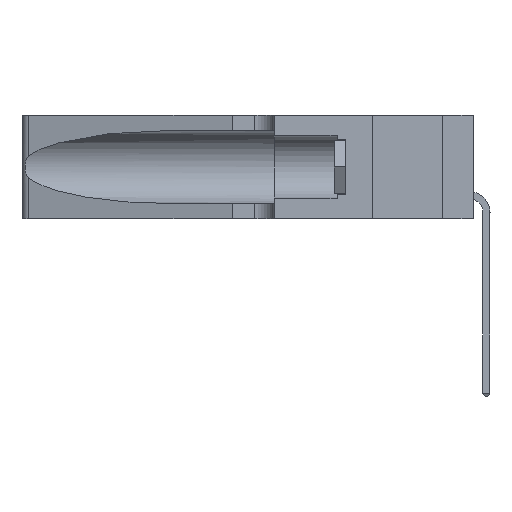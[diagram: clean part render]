
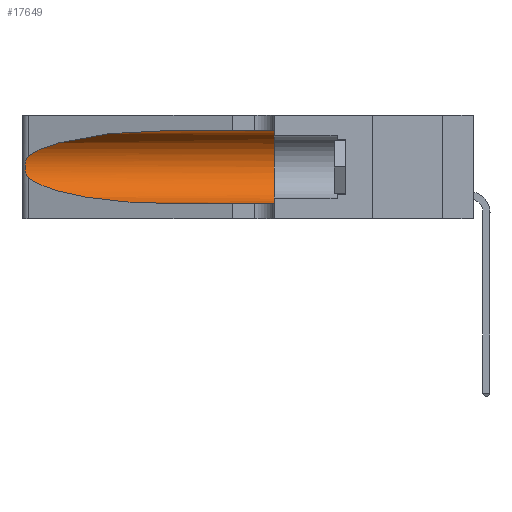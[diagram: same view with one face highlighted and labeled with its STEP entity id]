
A CAD part, left-side view. The second image highlights one B-rep face of the part: STEP entity #17649.
In plain terms, the highlighted cylindrical face has radius 3.308 mm (diameter 6.617 mm), a partial arc.
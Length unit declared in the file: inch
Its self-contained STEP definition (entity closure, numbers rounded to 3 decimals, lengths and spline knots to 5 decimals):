
#159 = DIRECTION ( 'NONE',  ( 0., -1., 0. ) ) ;
#1098 = CARTESIAN_POINT ( 'NONE',  ( 0.1305, 1.61858, 0.31525 ) ) ;
#1157 = FACE_OUTER_BOUND ( 'NONE', #19023, .T. ) ;
#1631 =( BOUNDED_CURVE ( )  B_SPLINE_CURVE ( 3, ( #22654, #5918, #21482, #34124 ),
 .UNSPECIFIED., .F., .F. ) 
 B_SPLINE_CURVE_WITH_KNOTS ( ( 4, 4 ),
 ( 1.5708, 2.84003 ),
 .UNSPECIFIED. ) 
 CURVE ( )  GEOMETRIC_REPRESENTATION_ITEM ( )  RATIONAL_B_SPLINE_CURVE ( ( 1., 0.87, 0.87, 1. ) ) 
 REPRESENTATION_ITEM ( '' )  );
#2338 = CARTESIAN_POINT ( 'NONE',  ( 0.25487, 1.22718, 0.14631 ) ) ;
#2506 = CARTESIAN_POINT ( 'NONE',  ( 0.25639, 1.23184, 0.21858 ) ) ;
#3030 = ORIENTED_EDGE ( 'NONE', *, *, #18477, .F. ) ;
#4092 = ORIENTED_EDGE ( 'NONE', *, *, #6124, .F. ) ;
#5155 =( BOUNDED_CURVE ( )  B_SPLINE_CURVE ( 3, ( #9189, #35853, #12946, #16282 ),
 .UNSPECIFIED., .F., .F. ) 
 B_SPLINE_CURVE_WITH_KNOTS ( ( 4, 4 ),
 ( 3.44316, 4.71239 ),
 .UNSPECIFIED. ) 
 CURVE ( )  GEOMETRIC_REPRESENTATION_ITEM ( )  RATIONAL_B_SPLINE_CURVE ( ( 1., 0.87, 0.87, 1. ) ) 
 REPRESENTATION_ITEM ( '' )  );
#5918 = CARTESIAN_POINT ( 'NONE',  ( 0.18966, 0.96281, 0.31525 ) ) ;
#6124 = EDGE_CURVE ( 'NONE', #10000, #37061, #9959, .T. ) ;
#6381 = CARTESIAN_POINT ( 'NONE',  ( 0.26075, 1.23896, 0.19203 ) ) ;
#6490 = VECTOR ( 'NONE', #39287, 39.37008 ) ;
#6588 = CARTESIAN_POINT ( 'NONE',  ( 0.1305, 0.72297, 0.05475 ) ) ;
#7759 = DIRECTION ( 'NONE',  ( 0., -1., 0. ) ) ;
#9189 = CARTESIAN_POINT ( 'NONE',  ( 0.25487, 1.22718, 0.14631 ) ) ;
#9807 = VERTEX_POINT ( 'NONE', #43419 ) ;
#9959 = CIRCLE ( 'NONE', #32583, 0.13025 ) ;
#10000 = VERTEX_POINT ( 'NONE', #25334 ) ;
#10020 = EDGE_CURVE ( 'NONE', #19557, #9807, #17262, .T. ) ;
#10081 = DIRECTION ( 'NONE',  ( 0., 0., 1. ) ) ;
#10137 = ORIENTED_EDGE ( 'NONE', *, *, #30398, .T. ) ;
#12946 = CARTESIAN_POINT ( 'NONE',  ( 0.18966, 0.96281, 0.05475 ) ) ;
#13775 = LINE ( 'NONE', #1098, #6490 ) ;
#15663 = VERTEX_POINT ( 'NONE', #6588 ) ;
#16282 = CARTESIAN_POINT ( 'NONE',  ( 0.1305, 0.72297, 0.05475 ) ) ;
#17262 = B_SPLINE_CURVE_WITH_KNOTS ( 'NONE', 3,
 ( #21267, #29200, #2506, #17743, #41362, #37626, #6381, #37298, #21608, #33735, #45384, #45232, #22258, #2338 ),
 .UNSPECIFIED., .F., .F.,
 ( 4, 2, 2, 2, 2, 2, 4 ),
 ( 0., 0.00027, 0.00053, 0.00107, 0.0016, 0.00187, 0.00214 ),
 .UNSPECIFIED. ) ;
#17649 = ADVANCED_FACE ( 'NONE', ( #1157 ), #28370, .F. ) ;
#17743 = CARTESIAN_POINT ( 'NONE',  ( 0.25787, 1.23484, 0.2124 ) ) ;
#18477 = EDGE_CURVE ( 'NONE', #38528, #10000, #13775, .T. ) ;
#19023 = EDGE_LOOP ( 'NONE', ( #20342, #33756, #35845, #10137, #4092, #3030 ) ) ;
#19557 = VERTEX_POINT ( 'NONE', #42575 ) ;
#20342 = ORIENTED_EDGE ( 'NONE', *, *, #35404, .T. ) ;
#21267 = CARTESIAN_POINT ( 'NONE',  ( 0.25487, 1.22718, 0.22369 ) ) ;
#21482 = CARTESIAN_POINT ( 'NONE',  ( 0.2373, 1.15595, 0.28018 ) ) ;
#21608 = CARTESIAN_POINT ( 'NONE',  ( 0.26017, 1.23833, 0.17102 ) ) ;
#22258 = CARTESIAN_POINT ( 'NONE',  ( 0.25555, 1.22993, 0.14849 ) ) ;
#22654 = CARTESIAN_POINT ( 'NONE',  ( 0.1305, 0.72297, 0.31525 ) ) ;
#23326 = CARTESIAN_POINT ( 'NONE',  ( 0.1305, 1.61858, 0.185 ) ) ;
#25334 = CARTESIAN_POINT ( 'NONE',  ( 0.1305, 0.35, 0.31525 ) ) ;
#28216 = AXIS2_PLACEMENT_3D ( 'NONE', #23326, #7759, #42233 ) ;
#28370 = CYLINDRICAL_SURFACE ( 'NONE', #28216, 0.13025 ) ;
#29200 = CARTESIAN_POINT ( 'NONE',  ( 0.25555, 1.22994, 0.2215 ) ) ;
#29816 = CARTESIAN_POINT ( 'NONE',  ( 0.1305, 0.35, 0.185 ) ) ;
#29987 = EDGE_CURVE ( 'NONE', #9807, #15663, #5155, .T. ) ;
#30398 = EDGE_CURVE ( 'NONE', #15663, #37061, #49797, .T. ) ;
#31693 = VECTOR ( 'NONE', #159, 39.37008 ) ;
#32583 = AXIS2_PLACEMENT_3D ( 'NONE', #29816, #37084, #10081 ) ;
#33735 = CARTESIAN_POINT ( 'NONE',  ( 0.25856, 1.23593, 0.16098 ) ) ;
#33756 = ORIENTED_EDGE ( 'NONE', *, *, #10020, .T. ) ;
#34124 = CARTESIAN_POINT ( 'NONE',  ( 0.25487, 1.22718, 0.22369 ) ) ;
#35404 = EDGE_CURVE ( 'NONE', #38528, #19557, #1631, .T. ) ;
#35845 = ORIENTED_EDGE ( 'NONE', *, *, #29987, .T. ) ;
#35853 = CARTESIAN_POINT ( 'NONE',  ( 0.2373, 1.15595, 0.08982 ) ) ;
#37061 = VERTEX_POINT ( 'NONE', #40590 ) ;
#37084 = DIRECTION ( 'NONE',  ( 0., 1., 0. ) ) ;
#37298 = CARTESIAN_POINT ( 'NONE',  ( 0.26075, 1.23896, 0.178 ) ) ;
#37626 = CARTESIAN_POINT ( 'NONE',  ( 0.26018, 1.23835, 0.19895 ) ) ;
#38528 = VERTEX_POINT ( 'NONE', #49964 ) ;
#39287 = DIRECTION ( 'NONE',  ( 0., -1., 0. ) ) ;
#40590 = CARTESIAN_POINT ( 'NONE',  ( 0.1305, 0.35, 0.05475 ) ) ;
#41362 = CARTESIAN_POINT ( 'NONE',  ( 0.25854, 1.2359, 0.20912 ) ) ;
#42233 = DIRECTION ( 'NONE',  ( 0., 0., -1. ) ) ;
#42575 = CARTESIAN_POINT ( 'NONE',  ( 0.25487, 1.22718, 0.22369 ) ) ;
#43419 = CARTESIAN_POINT ( 'NONE',  ( 0.25487, 1.22718, 0.14631 ) ) ;
#45232 = CARTESIAN_POINT ( 'NONE',  ( 0.25639, 1.23186, 0.15144 ) ) ;
#45384 = CARTESIAN_POINT ( 'NONE',  ( 0.25789, 1.23486, 0.15765 ) ) ;
#46435 = CARTESIAN_POINT ( 'NONE',  ( 0.1305, 1.61858, 0.05475 ) ) ;
#49797 = LINE ( 'NONE', #46435, #31693 ) ;
#49964 = CARTESIAN_POINT ( 'NONE',  ( 0.1305, 0.72297, 0.31525 ) ) ;
